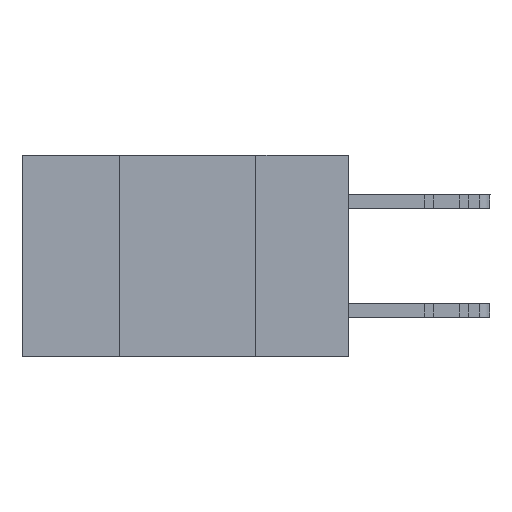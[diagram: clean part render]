
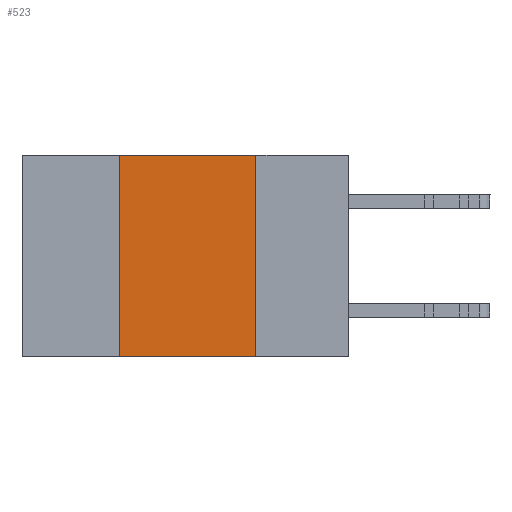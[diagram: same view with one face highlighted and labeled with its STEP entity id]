
A CAD part, left-side view. The second image highlights one B-rep face of the part: STEP entity #523.
In plain terms, the highlighted planar face has unit normal (-1, 0, 0).
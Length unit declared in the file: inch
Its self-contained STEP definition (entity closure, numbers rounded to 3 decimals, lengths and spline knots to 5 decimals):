
#523 = ADVANCED_FACE ( 'NONE', ( #31990 ), #9151, .F. ) ;
#1114 = CARTESIAN_POINT ( 'NONE',  ( 0., 0.17, 0. ) ) ;
#1961 = EDGE_CURVE ( 'NONE', #7600, #19909, #15435, .T. ) ;
#3750 = VERTEX_POINT ( 'NONE', #30277 ) ;
#3872 = DIRECTION ( 'NONE',  ( 0., 0., -1. ) ) ;
#4350 = EDGE_CURVE ( 'NONE', #3750, #8245, #18291, .T. ) ;
#4919 = LINE ( 'NONE', #30701, #19494 ) ;
#7600 = VERTEX_POINT ( 'NONE', #31802 ) ;
#7694 = DIRECTION ( 'NONE',  ( 0., 0., -1. ) ) ;
#7835 = CARTESIAN_POINT ( 'NONE',  ( 0., 0.6, -0.37 ) ) ;
#8216 = DIRECTION ( 'NONE',  ( 0., -1., 0. ) ) ;
#8245 = VERTEX_POINT ( 'NONE', #1114 ) ;
#9151 = PLANE ( 'NONE',  #29309 ) ;
#11737 = EDGE_LOOP ( 'NONE', ( #15601, #30269, #27193, #26158 ) ) ;
#14491 = CARTESIAN_POINT ( 'NONE',  ( 0., 0.17, -0.37 ) ) ;
#15142 = DIRECTION ( 'NONE',  ( 0., 0., 1. ) ) ;
#15435 = LINE ( 'NONE', #7835, #26248 ) ;
#15601 = ORIENTED_EDGE ( 'NONE', *, *, #16597, .F. ) ;
#16597 = EDGE_CURVE ( 'NONE', #8245, #19909, #22089, .T. ) ;
#17902 = DIRECTION ( 'NONE',  ( 0., -1., 0. ) ) ;
#18291 = LINE ( 'NONE', #23788, #24976 ) ;
#19494 = VECTOR ( 'NONE', #15142, 39.37008 ) ;
#19909 = VERTEX_POINT ( 'NONE', #14491 ) ;
#20052 = EDGE_CURVE ( 'NONE', #7600, #3750, #4919, .T. ) ;
#22089 = LINE ( 'NONE', #24924, #24765 ) ;
#23788 = CARTESIAN_POINT ( 'NONE',  ( 0., 0.6, 0. ) ) ;
#24560 = CARTESIAN_POINT ( 'NONE',  ( 0., 0.6, 0. ) ) ;
#24765 = VECTOR ( 'NONE', #7694, 39.37008 ) ;
#24924 = CARTESIAN_POINT ( 'NONE',  ( 0., 0.17, 0. ) ) ;
#24976 = VECTOR ( 'NONE', #8216, 39.37008 ) ;
#26158 = ORIENTED_EDGE ( 'NONE', *, *, #1961, .T. ) ;
#26248 = VECTOR ( 'NONE', #17902, 39.37008 ) ;
#27193 = ORIENTED_EDGE ( 'NONE', *, *, #20052, .F. ) ;
#29015 = DIRECTION ( 'NONE',  ( 1., 0., 0. ) ) ;
#29309 = AXIS2_PLACEMENT_3D ( 'NONE', #24560, #29015, #3872 ) ;
#30269 = ORIENTED_EDGE ( 'NONE', *, *, #4350, .F. ) ;
#30277 = CARTESIAN_POINT ( 'NONE',  ( 0., 0.42, 0. ) ) ;
#30701 = CARTESIAN_POINT ( 'NONE',  ( 0., 0.42, 0. ) ) ;
#31802 = CARTESIAN_POINT ( 'NONE',  ( 0., 0.42, -0.37 ) ) ;
#31990 = FACE_OUTER_BOUND ( 'NONE', #11737, .T. ) ;
